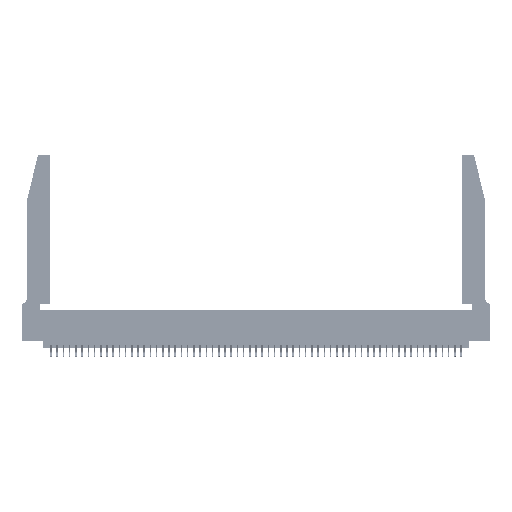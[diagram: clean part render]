
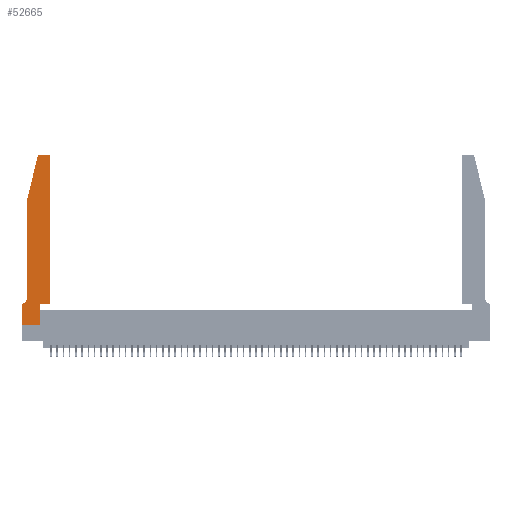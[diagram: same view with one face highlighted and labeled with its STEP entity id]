
A CAD part, top view. The second image highlights one B-rep face of the part: STEP entity #52665.
In plain terms, the highlighted planar face has unit normal (0, 0, 1).
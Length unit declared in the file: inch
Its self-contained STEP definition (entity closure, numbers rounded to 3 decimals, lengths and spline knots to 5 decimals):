
#17 = CARTESIAN_POINT ( 'NONE',  ( 0.2865, 0.35, 0.37 ) ) ;
#149 = EDGE_CURVE ( 'NONE', #17712, #37352, #48289, .T. ) ;
#319 = DIRECTION ( 'NONE',  ( 0., 0., 1. ) ) ;
#657 = LINE ( 'NONE', #22998, #45376 ) ;
#719 = VECTOR ( 'NONE', #9518, 39.37008 ) ;
#1767 = DIRECTION ( 'NONE',  ( -1., 0., 0. ) ) ;
#2079 = DIRECTION ( 'NONE',  ( 0., 0., 1. ) ) ;
#2536 = CARTESIAN_POINT ( 'NONE',  ( 0.4205, 2.75, 0.37 ) ) ;
#2666 = LINE ( 'NONE', #4174, #25214 ) ;
#4174 = CARTESIAN_POINT ( 'NONE',  ( 0.0755, 2., 0.37 ) ) ;
#4429 = DIRECTION ( 'NONE',  ( -1., 0., 0. ) ) ;
#5158 = DIRECTION ( 'NONE',  ( 0., 1., 0. ) ) ;
#5591 = EDGE_CURVE ( 'NONE', #27473, #27048, #14551, .T. ) ;
#6077 = CARTESIAN_POINT ( 'NONE',  ( 0.2865, 0.35, 0.37 ) ) ;
#6142 = VECTOR ( 'NONE', #45274, 39.37008 ) ;
#7134 = EDGE_CURVE ( 'NONE', #12103, #15814, #15771, .T. ) ;
#7613 = CARTESIAN_POINT ( 'NONE',  ( 0.4505, 2.72, 0.37 ) ) ;
#7881 = ORIENTED_EDGE ( 'NONE', *, *, #19437, .T. ) ;
#7954 = VECTOR ( 'NONE', #5158, 39.37008 ) ;
#8613 = LINE ( 'NONE', #50374, #17234 ) ;
#9518 = DIRECTION ( 'NONE',  ( 1., 0., 0. ) ) ;
#10199 = EDGE_CURVE ( 'NONE', #33518, #12103, #24632, .T. ) ;
#10895 = CARTESIAN_POINT ( 'NONE',  ( 0.25487, 2.72718, 0.37 ) ) ;
#11680 = CARTESIAN_POINT ( 'NONE',  ( 0.4205, 2.72, 0.37 ) ) ;
#11896 = CARTESIAN_POINT ( 'NONE',  ( 0.0755, 2., 0.37 ) ) ;
#12103 = VERTEX_POINT ( 'NONE', #12377 ) ;
#12377 = CARTESIAN_POINT ( 'NONE',  ( 0.2865, 0., 0.37 ) ) ;
#12897 = CARTESIAN_POINT ( 'NONE',  ( 0.0055, 0.35, 0.37 ) ) ;
#13237 = ORIENTED_EDGE ( 'NONE', *, *, #149, .T. ) ;
#13244 = CARTESIAN_POINT ( 'NONE',  ( 0.284, 2.75, 0.37 ) ) ;
#13694 = CARTESIAN_POINT ( 'NONE',  ( 0.0755, 0.42, 0.37 ) ) ;
#13924 = VECTOR ( 'NONE', #41166, 39.37008 ) ;
#14551 = CIRCLE ( 'NONE', #42711, 0.03 ) ;
#14589 = ORIENTED_EDGE ( 'NONE', *, *, #7134, .T. ) ;
#15771 = LINE ( 'NONE', #17, #47741 ) ;
#15814 = VERTEX_POINT ( 'NONE', #6077 ) ;
#15939 = DIRECTION ( 'NONE',  ( 1., 0., 0. ) ) ;
#17210 = CARTESIAN_POINT ( 'NONE',  ( 0.0755, 2., 0.37 ) ) ;
#17234 = VECTOR ( 'NONE', #4429, 39.37008 ) ;
#17712 = VERTEX_POINT ( 'NONE', #13694 ) ;
#17838 = ORIENTED_EDGE ( 'NONE', *, *, #28462, .T. ) ;
#19030 = ORIENTED_EDGE ( 'NONE', *, *, #49699, .T. ) ;
#19437 = EDGE_CURVE ( 'NONE', #43907, #32140, #28868, .T. ) ;
#22603 = EDGE_CURVE ( 'NONE', #15814, #24860, #657, .T. ) ;
#22998 = CARTESIAN_POINT ( 'NONE',  ( 0.4505, 0.35, 0.37 ) ) ;
#24632 = LINE ( 'NONE', #38835, #719 ) ;
#24860 = VERTEX_POINT ( 'NONE', #32549 ) ;
#25214 = VECTOR ( 'NONE', #33683, 39.37008 ) ;
#25763 = PLANE ( 'NONE',  #28446 ) ;
#27048 = VERTEX_POINT ( 'NONE', #10895 ) ;
#27181 = DIRECTION ( 'NONE',  ( 0., 0., -1. ) ) ;
#27473 = VERTEX_POINT ( 'NONE', #13244 ) ;
#27485 = CARTESIAN_POINT ( 'NONE',  ( 0.284, 2.72, 0.37 ) ) ;
#28109 = FACE_OUTER_BOUND ( 'NONE', #50622, .T. ) ;
#28209 = AXIS2_PLACEMENT_3D ( 'NONE', #11680, #40948, #15939 ) ;
#28446 = AXIS2_PLACEMENT_3D ( 'NONE', #50600, #319, #29970 ) ;
#28462 = EDGE_CURVE ( 'NONE', #43602, #33518, #38320, .T. ) ;
#28868 = CIRCLE ( 'NONE', #28209, 0.03 ) ;
#29109 = ORIENTED_EDGE ( 'NONE', *, *, #5591, .T. ) ;
#29970 = DIRECTION ( 'NONE',  ( 1., 0., 0. ) ) ;
#30458 = CARTESIAN_POINT ( 'NONE',  ( 0.4505, 0.35, 0.37 ) ) ;
#31054 = ORIENTED_EDGE ( 'NONE', *, *, #31677, .T. ) ;
#31504 = ORIENTED_EDGE ( 'NONE', *, *, #22603, .T. ) ;
#31677 = EDGE_CURVE ( 'NONE', #37352, #43602, #51270, .T. ) ;
#31705 = DIRECTION ( 'NONE',  ( 1., 0., 0. ) ) ;
#32140 = VERTEX_POINT ( 'NONE', #2536 ) ;
#32549 = CARTESIAN_POINT ( 'NONE',  ( 0.4505, 0.35, 0.37 ) ) ;
#33518 = VERTEX_POINT ( 'NONE', #45003 ) ;
#33683 = DIRECTION ( 'NONE',  ( 0., -1., 0. ) ) ;
#34929 = LINE ( 'NONE', #11896, #13924 ) ;
#34933 = ORIENTED_EDGE ( 'NONE', *, *, #41968, .T. ) ;
#34966 = AXIS2_PLACEMENT_3D ( 'NONE', #52033, #27181, #1767 ) ;
#36241 = ORIENTED_EDGE ( 'NONE', *, *, #48193, .T. ) ;
#37352 = VERTEX_POINT ( 'NONE', #12897 ) ;
#38320 = LINE ( 'NONE', #41109, #6142 ) ;
#38835 = CARTESIAN_POINT ( 'NONE',  ( 0., 0., 0.37 ) ) ;
#39572 = CARTESIAN_POINT ( 'NONE',  ( 0., 0.35, 0.37 ) ) ;
#40948 = DIRECTION ( 'NONE',  ( 0., 0., 1. ) ) ;
#41109 = CARTESIAN_POINT ( 'NONE',  ( 0., 0., 0.37 ) ) ;
#41166 = DIRECTION ( 'NONE',  ( -0.239, -0.971, 0. ) ) ;
#41376 = CARTESIAN_POINT ( 'NONE',  ( 0.0755, 0.35, 0.37 ) ) ;
#41968 = EDGE_CURVE ( 'NONE', #27048, #44353, #34929, .T. ) ;
#42139 = EDGE_CURVE ( 'NONE', #32140, #27473, #8613, .T. ) ;
#42711 = AXIS2_PLACEMENT_3D ( 'NONE', #27485, #2079, #31705 ) ;
#43602 = VERTEX_POINT ( 'NONE', #39572 ) ;
#43907 = VERTEX_POINT ( 'NONE', #7613 ) ;
#44353 = VERTEX_POINT ( 'NONE', #17210 ) ;
#45003 = CARTESIAN_POINT ( 'NONE',  ( 0., 0., 0.37 ) ) ;
#45274 = DIRECTION ( 'NONE',  ( 0., -1., 0. ) ) ;
#45376 = VECTOR ( 'NONE', #52110, 39.37008 ) ;
#47741 = VECTOR ( 'NONE', #50520, 39.37008 ) ;
#48193 = EDGE_CURVE ( 'NONE', #44353, #17712, #2666, .T. ) ;
#48289 = CIRCLE ( 'NONE', #34966, 0.07 ) ;
#49699 = EDGE_CURVE ( 'NONE', #24860, #43907, #49803, .T. ) ;
#49803 = LINE ( 'NONE', #30458, #7954 ) ;
#49817 = ORIENTED_EDGE ( 'NONE', *, *, #42139, .T. ) ;
#49870 = DIRECTION ( 'NONE',  ( -1., 0., 0. ) ) ;
#49948 = VECTOR ( 'NONE', #49870, 39.37008 ) ;
#50374 = CARTESIAN_POINT ( 'NONE',  ( 0.2605, 2.75, 0.37 ) ) ;
#50520 = DIRECTION ( 'NONE',  ( 0., 1., 0. ) ) ;
#50600 = CARTESIAN_POINT ( 'NONE',  ( 0., 0.35, 0.37 ) ) ;
#50622 = EDGE_LOOP ( 'NONE', ( #49817, #29109, #34933, #36241, #13237, #31054, #17838, #52407, #14589, #31504, #19030, #7881 ) ) ;
#51270 = LINE ( 'NONE', #41376, #49948 ) ;
#52033 = CARTESIAN_POINT ( 'NONE',  ( 0.0055, 0.42, 0.37 ) ) ;
#52110 = DIRECTION ( 'NONE',  ( 1., 0., 0. ) ) ;
#52407 = ORIENTED_EDGE ( 'NONE', *, *, #10199, .T. ) ;
#52665 = ADVANCED_FACE ( 'NONE', ( #28109 ), #25763, .T. ) ;
